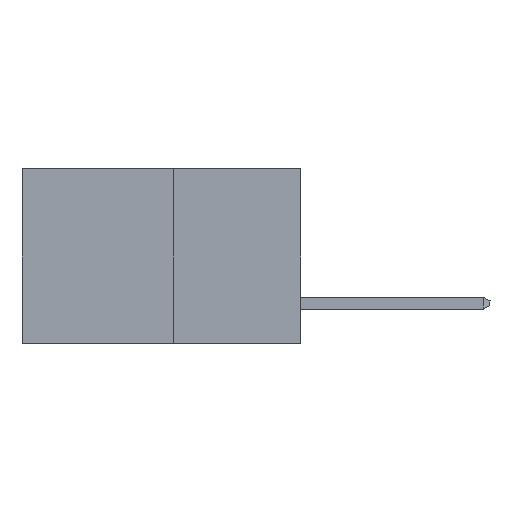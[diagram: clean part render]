
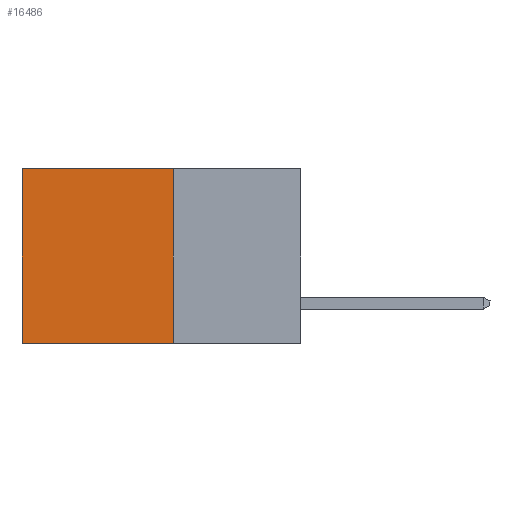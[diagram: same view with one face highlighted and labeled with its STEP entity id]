
A CAD part, left-side view. The second image highlights one B-rep face of the part: STEP entity #16486.
In plain terms, the highlighted planar face has unit normal (-1, 0, 0).
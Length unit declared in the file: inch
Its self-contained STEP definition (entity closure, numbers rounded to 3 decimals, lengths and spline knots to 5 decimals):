
#190 = CARTESIAN_POINT ( 'NONE',  ( 0.277, 0.27, -0.37 ) ) ;
#407 = ORIENTED_EDGE ( 'NONE', *, *, #11827, .T. ) ;
#481 = EDGE_LOOP ( 'NONE', ( #407, #10265, #12253, #9729 ) ) ;
#1082 = CARTESIAN_POINT ( 'NONE',  ( 0.277, 0.59, 0. ) ) ;
#2033 = AXIS2_PLACEMENT_3D ( 'NONE', #190, #12480, #4341 ) ;
#2395 = VECTOR ( 'NONE', #17042, 39.37008 ) ;
#3401 = CARTESIAN_POINT ( 'NONE',  ( 0.277, 0.59, -0.37 ) ) ;
#3886 = VERTEX_POINT ( 'NONE', #9899 ) ;
#4341 = DIRECTION ( 'NONE',  ( 0., 0., -1. ) ) ;
#4564 = LINE ( 'NONE', #7395, #9533 ) ;
#4660 = VERTEX_POINT ( 'NONE', #10173 ) ;
#5145 = LINE ( 'NONE', #8191, #14706 ) ;
#5470 = DIRECTION ( 'NONE',  ( 0., 1., 0. ) ) ;
#6097 = LINE ( 'NONE', #14340, #2395 ) ;
#6844 = FACE_OUTER_BOUND ( 'NONE', #481, .T. ) ;
#7325 = EDGE_CURVE ( 'NONE', #3886, #12061, #5145, .T. ) ;
#7395 = CARTESIAN_POINT ( 'NONE',  ( 0.277, 0.27, 0. ) ) ;
#8191 = CARTESIAN_POINT ( 'NONE',  ( 0.277, 0.27, -0.37 ) ) ;
#9190 = LINE ( 'NONE', #13760, #11903 ) ;
#9533 = VECTOR ( 'NONE', #16823, 39.37008 ) ;
#9729 = ORIENTED_EDGE ( 'NONE', *, *, #14002, .T. ) ;
#9802 = DIRECTION ( 'NONE',  ( 0., 0., -1. ) ) ;
#9899 = CARTESIAN_POINT ( 'NONE',  ( 0.277, 0.27, -0.37 ) ) ;
#10173 = CARTESIAN_POINT ( 'NONE',  ( 0.277, 0.27, 0. ) ) ;
#10265 = ORIENTED_EDGE ( 'NONE', *, *, #7325, .F. ) ;
#11827 = EDGE_CURVE ( 'NONE', #15555, #12061, #9190, .T. ) ;
#11903 = VECTOR ( 'NONE', #9802, 39.37008 ) ;
#12061 = VERTEX_POINT ( 'NONE', #3401 ) ;
#12253 = ORIENTED_EDGE ( 'NONE', *, *, #14135, .F. ) ;
#12480 = DIRECTION ( 'NONE',  ( 1., 0., 0. ) ) ;
#13760 = CARTESIAN_POINT ( 'NONE',  ( 0.277, 0.59, -0.37 ) ) ;
#14002 = EDGE_CURVE ( 'NONE', #4660, #15555, #4564, .T. ) ;
#14135 = EDGE_CURVE ( 'NONE', #4660, #3886, #6097, .T. ) ;
#14340 = CARTESIAN_POINT ( 'NONE',  ( 0.277, 0.27, -0.37 ) ) ;
#14706 = VECTOR ( 'NONE', #5470, 39.37008 ) ;
#15555 = VERTEX_POINT ( 'NONE', #1082 ) ;
#16486 = ADVANCED_FACE ( 'NONE', ( #6844 ), #16510, .F. ) ;
#16510 = PLANE ( 'NONE',  #2033 ) ;
#16823 = DIRECTION ( 'NONE',  ( 0., 1., 0. ) ) ;
#17042 = DIRECTION ( 'NONE',  ( 0., 0., -1. ) ) ;
